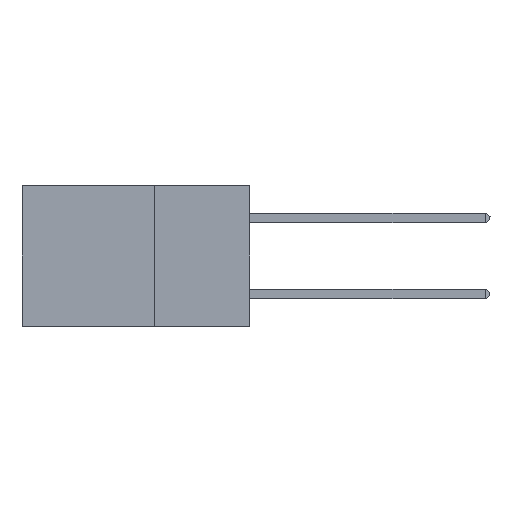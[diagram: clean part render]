
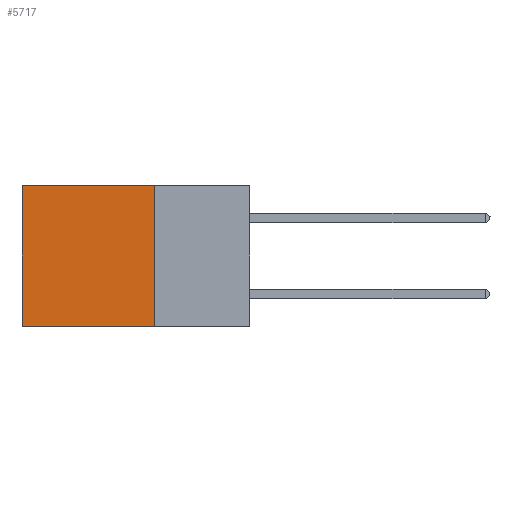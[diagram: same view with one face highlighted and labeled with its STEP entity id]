
A CAD part, left-side view. The second image highlights one B-rep face of the part: STEP entity #5717.
In plain terms, the highlighted planar face has unit normal (-1, 0, 0).
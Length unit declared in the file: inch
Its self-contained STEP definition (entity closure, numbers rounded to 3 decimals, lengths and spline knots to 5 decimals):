
#342 = LINE ( 'NONE', #5039, #9848 ) ;
#846 = ORIENTED_EDGE ( 'NONE', *, *, #10036, .T. ) ;
#1504 = VECTOR ( 'NONE', #1871, 39.37008 ) ;
#1871 = DIRECTION ( 'NONE',  ( 0., 0., -1. ) ) ;
#2078 = DIRECTION ( 'NONE',  ( 0., 1., 0. ) ) ;
#2092 = ORIENTED_EDGE ( 'NONE', *, *, #7330, .T. ) ;
#2210 = VERTEX_POINT ( 'NONE', #5928 ) ;
#3024 = LINE ( 'NONE', #13361, #1504 ) ;
#3106 = DIRECTION ( 'NONE',  ( 0., 0., -1. ) ) ;
#4494 = VECTOR ( 'NONE', #9740, 39.37008 ) ;
#4628 = VERTEX_POINT ( 'NONE', #9644 ) ;
#5039 = CARTESIAN_POINT ( 'NONE',  ( 0.2875, 0.6, 0. ) ) ;
#5129 = ORIENTED_EDGE ( 'NONE', *, *, #6119, .F. ) ;
#5513 = FACE_OUTER_BOUND ( 'NONE', #6569, .T. ) ;
#5717 = ADVANCED_FACE ( 'NONE', ( #5513 ), #14907, .F. ) ;
#5928 = CARTESIAN_POINT ( 'NONE',  ( 0.2875, 0.6, -0.37 ) ) ;
#6119 = EDGE_CURVE ( 'NONE', #4628, #12137, #3024, .T. ) ;
#6298 = ORIENTED_EDGE ( 'NONE', *, *, #13214, .F. ) ;
#6569 = EDGE_LOOP ( 'NONE', ( #2092, #6298, #5129, #846 ) ) ;
#6980 = VERTEX_POINT ( 'NONE', #11461 ) ;
#7330 = EDGE_CURVE ( 'NONE', #6980, #2210, #342, .T. ) ;
#8810 = LINE ( 'NONE', #9974, #4494 ) ;
#9135 = CARTESIAN_POINT ( 'NONE',  ( 0.2875, 0.25, 0. ) ) ;
#9644 = CARTESIAN_POINT ( 'NONE',  ( 0.2875, 0.25, 0. ) ) ;
#9724 = DIRECTION ( 'NONE',  ( 0., 0., -1. ) ) ;
#9740 = DIRECTION ( 'NONE',  ( 0., 1., 0. ) ) ;
#9848 = VECTOR ( 'NONE', #9724, 39.37008 ) ;
#9974 = CARTESIAN_POINT ( 'NONE',  ( 0.2875, 0.25, 0. ) ) ;
#10036 = EDGE_CURVE ( 'NONE', #4628, #6980, #8810, .T. ) ;
#11461 = CARTESIAN_POINT ( 'NONE',  ( 0.2875, 0.6, 0. ) ) ;
#11567 = LINE ( 'NONE', #12630, #14935 ) ;
#12137 = VERTEX_POINT ( 'NONE', #14173 ) ;
#12630 = CARTESIAN_POINT ( 'NONE',  ( 0.2875, 0.25, -0.37 ) ) ;
#12748 = DIRECTION ( 'NONE',  ( 1., 0., 0. ) ) ;
#13214 = EDGE_CURVE ( 'NONE', #12137, #2210, #11567, .T. ) ;
#13361 = CARTESIAN_POINT ( 'NONE',  ( 0.2875, 0.25, 0. ) ) ;
#14173 = CARTESIAN_POINT ( 'NONE',  ( 0.2875, 0.25, -0.37 ) ) ;
#14907 = PLANE ( 'NONE',  #14976 ) ;
#14935 = VECTOR ( 'NONE', #2078, 39.37008 ) ;
#14976 = AXIS2_PLACEMENT_3D ( 'NONE', #9135, #12748, #3106 ) ;
